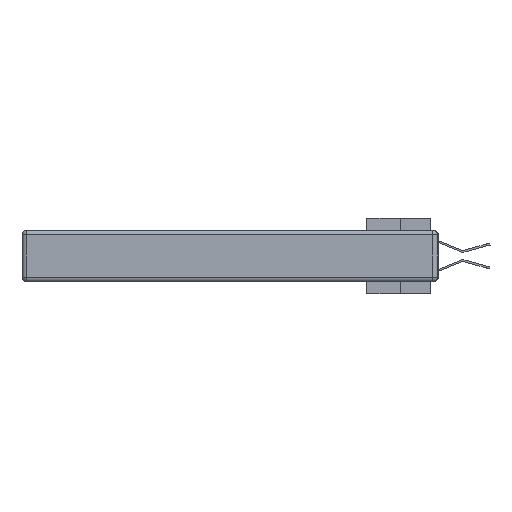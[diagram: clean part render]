
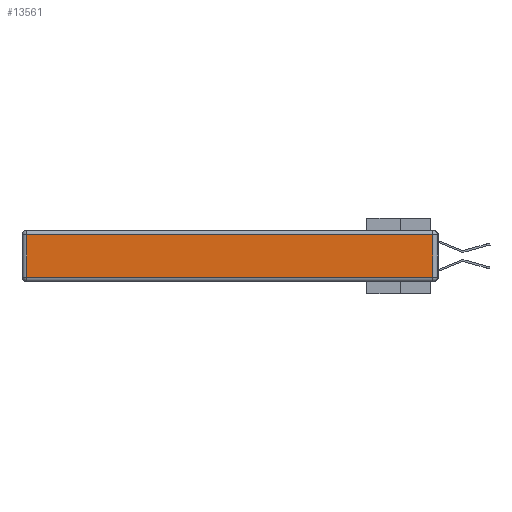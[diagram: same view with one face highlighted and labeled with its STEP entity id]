
A CAD part, left-side view. The second image highlights one B-rep face of the part: STEP entity #13561.
In plain terms, the highlighted planar face has unit normal (-1, 0, 0).
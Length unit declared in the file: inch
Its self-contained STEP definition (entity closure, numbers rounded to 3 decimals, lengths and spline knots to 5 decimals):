
#209 = VECTOR ( 'NONE', #24943, 39.37008 ) ;
#288 = CARTESIAN_POINT ( 'NONE',  ( 0., 0., -0.343 ) ) ;
#3621 = CARTESIAN_POINT ( 'NONE',  ( 0., 2.72, -0.313 ) ) ;
#4311 = VECTOR ( 'NONE', #32116, 39.37008 ) ;
#5133 = CARTESIAN_POINT ( 'NONE',  ( 0., 2.75, -0.03 ) ) ;
#7886 = VERTEX_POINT ( 'NONE', #17575 ) ;
#7913 = CARTESIAN_POINT ( 'NONE',  ( 0., 2.72, -0.343 ) ) ;
#9863 = AXIS2_PLACEMENT_3D ( 'NONE', #288, #11965, #18132 ) ;
#9975 = DIRECTION ( 'NONE',  ( 0., -1., 0. ) ) ;
#11842 = VERTEX_POINT ( 'NONE', #28560 ) ;
#11965 = DIRECTION ( 'NONE',  ( -1., 0., 0. ) ) ;
#13561 = ADVANCED_FACE ( 'NONE', ( #32741 ), #26622, .T. ) ;
#13754 = EDGE_CURVE ( 'NONE', #7886, #26379, #16959, .T. ) ;
#14056 = EDGE_CURVE ( 'NONE', #11842, #7886, #16286, .T. ) ;
#14210 = ORIENTED_EDGE ( 'NONE', *, *, #20878, .T. ) ;
#15861 = EDGE_LOOP ( 'NONE', ( #14210, #37115, #20265, #29924 ) ) ;
#16286 = LINE ( 'NONE', #5133, #31040 ) ;
#16900 = CARTESIAN_POINT ( 'NONE',  ( 0., 0.03, -0.313 ) ) ;
#16959 = LINE ( 'NONE', #7913, #4311 ) ;
#17575 = CARTESIAN_POINT ( 'NONE',  ( 0., 2.72, -0.03 ) ) ;
#18132 = DIRECTION ( 'NONE',  ( 0., 0., 1. ) ) ;
#20265 = ORIENTED_EDGE ( 'NONE', *, *, #14056, .T. ) ;
#20878 = EDGE_CURVE ( 'NONE', #26379, #20959, #27500, .T. ) ;
#20959 = VERTEX_POINT ( 'NONE', #16900 ) ;
#21939 = CARTESIAN_POINT ( 'NONE',  ( 0., 0., -0.313 ) ) ;
#22072 = CARTESIAN_POINT ( 'NONE',  ( 0., 0.03, -0.343 ) ) ;
#24379 = LINE ( 'NONE', #22072, #209 ) ;
#24943 = DIRECTION ( 'NONE',  ( 0., 0., 1. ) ) ;
#26379 = VERTEX_POINT ( 'NONE', #3621 ) ;
#26622 = PLANE ( 'NONE',  #9863 ) ;
#27500 = LINE ( 'NONE', #21939, #33177 ) ;
#28560 = CARTESIAN_POINT ( 'NONE',  ( 0., 0.03, -0.03 ) ) ;
#29924 = ORIENTED_EDGE ( 'NONE', *, *, #13754, .T. ) ;
#31040 = VECTOR ( 'NONE', #33775, 39.37008 ) ;
#32116 = DIRECTION ( 'NONE',  ( 0., 0., -1. ) ) ;
#32741 = FACE_OUTER_BOUND ( 'NONE', #15861, .T. ) ;
#33177 = VECTOR ( 'NONE', #9975, 39.37008 ) ;
#33775 = DIRECTION ( 'NONE',  ( 0., 1., 0. ) ) ;
#35999 = EDGE_CURVE ( 'NONE', #20959, #11842, #24379, .T. ) ;
#37115 = ORIENTED_EDGE ( 'NONE', *, *, #35999, .T. ) ;
